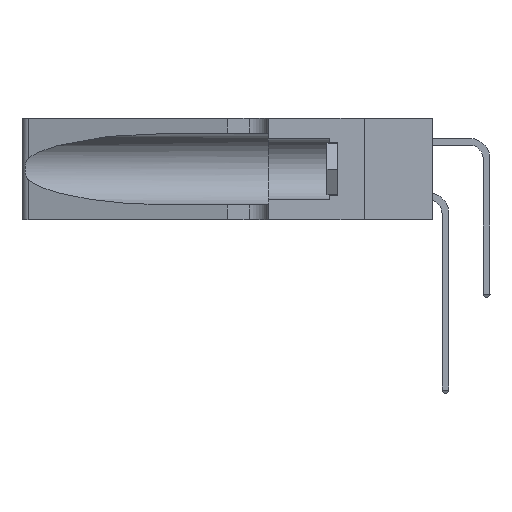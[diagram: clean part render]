
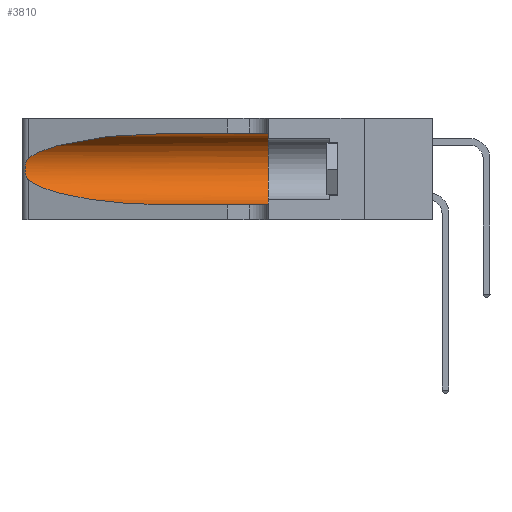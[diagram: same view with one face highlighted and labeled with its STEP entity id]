
A CAD part, left-side view. The second image highlights one B-rep face of the part: STEP entity #3810.
In plain terms, the highlighted cylindrical face has radius 3.308 mm (diameter 6.617 mm), a partial arc.
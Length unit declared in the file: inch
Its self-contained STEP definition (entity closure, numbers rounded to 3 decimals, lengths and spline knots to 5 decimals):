
#267 = CARTESIAN_POINT ( 'NONE',  ( 0.1305, 0.72297, 0.05475 ) ) ;
#531 =( BOUNDED_CURVE ( )  B_SPLINE_CURVE ( 3, ( #4629, #9298, #9353, #3007 ),
 .UNSPECIFIED., .F., .T. ) 
 B_SPLINE_CURVE_WITH_KNOTS ( ( 4, 4 ),
 ( 1.5708, 2.84003 ),
 .UNSPECIFIED. ) 
 CURVE ( )  GEOMETRIC_REPRESENTATION_ITEM ( )  RATIONAL_B_SPLINE_CURVE ( ( 1., 0.87, 0.87, 1. ) ) 
 REPRESENTATION_ITEM ( '' )  );
#634 = CARTESIAN_POINT ( 'NONE',  ( 0.1305, 0.72297, 0.05475 ) ) ;
#1257 = CARTESIAN_POINT ( 'NONE',  ( 0.26017, 1.23833, 0.17102 ) ) ;
#2501 = VERTEX_POINT ( 'NONE', #634 ) ;
#2660 = CARTESIAN_POINT ( 'NONE',  ( 0.25487, 1.22718, 0.22369 ) ) ;
#2734 = CARTESIAN_POINT ( 'NONE',  ( 0.25789, 1.23486, 0.15765 ) ) ;
#3007 = CARTESIAN_POINT ( 'NONE',  ( 0.25487, 1.22718, 0.22369 ) ) ;
#3058 = DIRECTION ( 'NONE',  ( 0., 0., 1. ) ) ;
#3414 = ORIENTED_EDGE ( 'NONE', *, *, #5868, .T. ) ;
#3810 = ADVANCED_FACE ( 'NONE', ( #16592 ), #14558, .F. ) ;
#3947 = CARTESIAN_POINT ( 'NONE',  ( 0.1305, 1.61858, 0.185 ) ) ;
#4147 = CARTESIAN_POINT ( 'NONE',  ( 0.25854, 1.2359, 0.20912 ) ) ;
#4186 = CARTESIAN_POINT ( 'NONE',  ( 0.1305, 1.61858, 0.31525 ) ) ;
#4225 = CARTESIAN_POINT ( 'NONE',  ( 0.25856, 1.23593, 0.16098 ) ) ;
#4290 = CARTESIAN_POINT ( 'NONE',  ( 0.25787, 1.23484, 0.2124 ) ) ;
#4370 = VECTOR ( 'NONE', #14844, 39.37008 ) ;
#4434 = CARTESIAN_POINT ( 'NONE',  ( 0.1305, 0.35, 0.185 ) ) ;
#4541 = AXIS2_PLACEMENT_3D ( 'NONE', #3947, #7171, #19465 ) ;
#4629 = CARTESIAN_POINT ( 'NONE',  ( 0.1305, 0.72297, 0.31525 ) ) ;
#5522 = CARTESIAN_POINT ( 'NONE',  ( 0.25487, 1.22718, 0.14631 ) ) ;
#5629 = LINE ( 'NONE', #4186, #17393 ) ;
#5737 = DIRECTION ( 'NONE',  ( 0., -1., 0. ) ) ;
#5781 = CARTESIAN_POINT ( 'NONE',  ( 0.25639, 1.23184, 0.21858 ) ) ;
#5868 = EDGE_CURVE ( 'NONE', #10336, #2501, #11168, .T. ) ;
#6106 = AXIS2_PLACEMENT_3D ( 'NONE', #4434, #15185, #3058 ) ;
#6245 = VERTEX_POINT ( 'NONE', #18143 ) ;
#6462 = EDGE_CURVE ( 'NONE', #2501, #6245, #8473, .T. ) ;
#6505 = VERTEX_POINT ( 'NONE', #16553 ) ;
#7171 = DIRECTION ( 'NONE',  ( 0., -1., 0. ) ) ;
#7425 = CARTESIAN_POINT ( 'NONE',  ( 0.25487, 1.22718, 0.14631 ) ) ;
#8095 = CARTESIAN_POINT ( 'NONE',  ( 0.25487, 1.22718, 0.14631 ) ) ;
#8277 = ORIENTED_EDGE ( 'NONE', *, *, #13194, .F. ) ;
#8473 = LINE ( 'NONE', #13315, #4370 ) ;
#9298 = CARTESIAN_POINT ( 'NONE',  ( 0.18966, 0.96281, 0.31525 ) ) ;
#9353 = CARTESIAN_POINT ( 'NONE',  ( 0.2373, 1.15595, 0.28018 ) ) ;
#9796 = ORIENTED_EDGE ( 'NONE', *, *, #6462, .T. ) ;
#10175 = EDGE_LOOP ( 'NONE', ( #19846, #16977, #3414, #9796, #13666, #8277 ) ) ;
#10326 = CARTESIAN_POINT ( 'NONE',  ( 0.25555, 1.22994, 0.2215 ) ) ;
#10336 = VERTEX_POINT ( 'NONE', #5522 ) ;
#11168 =( BOUNDED_CURVE ( )  B_SPLINE_CURVE ( 3, ( #8095, #14252, #15606, #267 ),
 .UNSPECIFIED., .F., .T. ) 
 B_SPLINE_CURVE_WITH_KNOTS ( ( 4, 4 ),
 ( 3.44316, 4.71239 ),
 .UNSPECIFIED. ) 
 CURVE ( )  GEOMETRIC_REPRESENTATION_ITEM ( )  RATIONAL_B_SPLINE_CURVE ( ( 1., 0.87, 0.87, 1. ) ) 
 REPRESENTATION_ITEM ( '' )  );
#11195 = EDGE_CURVE ( 'NONE', #19226, #17566, #531, .T. ) ;
#11850 = CARTESIAN_POINT ( 'NONE',  ( 0.26075, 1.23896, 0.19203 ) ) ;
#13194 = EDGE_CURVE ( 'NONE', #19226, #6505, #5629, .T. ) ;
#13315 = CARTESIAN_POINT ( 'NONE',  ( 0.1305, 1.61858, 0.05475 ) ) ;
#13398 = CARTESIAN_POINT ( 'NONE',  ( 0.26075, 1.23896, 0.178 ) ) ;
#13583 = CARTESIAN_POINT ( 'NONE',  ( 0.25555, 1.22993, 0.14849 ) ) ;
#13666 = ORIENTED_EDGE ( 'NONE', *, *, #14120, .F. ) ;
#14120 = EDGE_CURVE ( 'NONE', #6505, #6245, #14470, .T. ) ;
#14252 = CARTESIAN_POINT ( 'NONE',  ( 0.2373, 1.15595, 0.08982 ) ) ;
#14470 = CIRCLE ( 'NONE', #6106, 0.13025 ) ;
#14558 = CYLINDRICAL_SURFACE ( 'NONE', #4541, 0.13025 ) ;
#14844 = DIRECTION ( 'NONE',  ( 0., -1., 0. ) ) ;
#15185 = DIRECTION ( 'NONE',  ( 0., 1., 0. ) ) ;
#15606 = CARTESIAN_POINT ( 'NONE',  ( 0.18966, 0.96281, 0.05475 ) ) ;
#16553 = CARTESIAN_POINT ( 'NONE',  ( 0.1305, 0.35, 0.31525 ) ) ;
#16560 = CARTESIAN_POINT ( 'NONE',  ( 0.1305, 0.72297, 0.31525 ) ) ;
#16592 = FACE_OUTER_BOUND ( 'NONE', #10175, .T. ) ;
#16620 = CARTESIAN_POINT ( 'NONE',  ( 0.25639, 1.23186, 0.15144 ) ) ;
#16977 = ORIENTED_EDGE ( 'NONE', *, *, #19221, .T. ) ;
#17393 = VECTOR ( 'NONE', #5737, 39.37008 ) ;
#17566 = VERTEX_POINT ( 'NONE', #19112 ) ;
#18143 = CARTESIAN_POINT ( 'NONE',  ( 0.1305, 0.35, 0.05475 ) ) ;
#19112 = CARTESIAN_POINT ( 'NONE',  ( 0.25487, 1.22718, 0.22369 ) ) ;
#19221 = EDGE_CURVE ( 'NONE', #17566, #10336, #19621, .T. ) ;
#19226 = VERTEX_POINT ( 'NONE', #16560 ) ;
#19459 = CARTESIAN_POINT ( 'NONE',  ( 0.26018, 1.23835, 0.19895 ) ) ;
#19465 = DIRECTION ( 'NONE',  ( 0., 0., -1. ) ) ;
#19621 = B_SPLINE_CURVE_WITH_KNOTS ( 'NONE', 3,
 ( #2660, #10326, #5781, #4290, #4147, #19459, #11850, #13398, #1257, #4225, #2734, #16620, #13583, #7425 ),
 .UNSPECIFIED., .F., .F.,
 ( 4, 2, 2, 2, 2, 2, 4 ),
 ( 0., 0.00027, 0.00053, 0.00107, 0.0016, 0.00187, 0.00214 ),
 .UNSPECIFIED. ) ;
#19846 = ORIENTED_EDGE ( 'NONE', *, *, #11195, .T. ) ;
